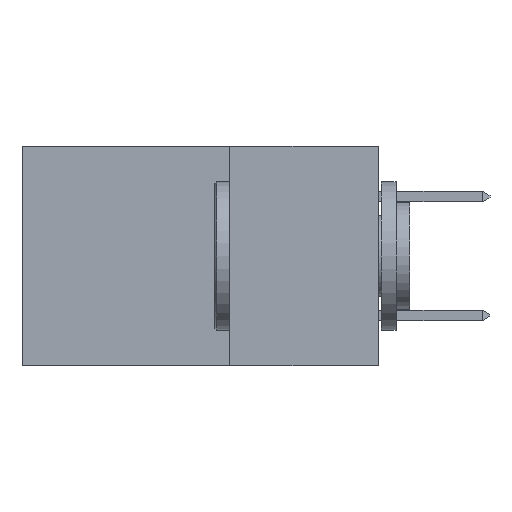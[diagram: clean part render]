
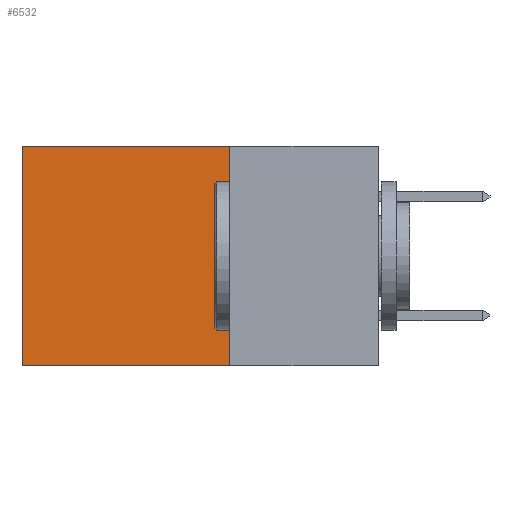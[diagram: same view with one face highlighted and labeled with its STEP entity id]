
A CAD part, left-side view. The second image highlights one B-rep face of the part: STEP entity #6532.
In plain terms, the highlighted planar face has unit normal (-1, 0, 0).
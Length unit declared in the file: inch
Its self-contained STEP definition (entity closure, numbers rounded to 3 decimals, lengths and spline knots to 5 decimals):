
#252 = LINE ( 'NONE', #10762, #7019 ) ;
#989 = EDGE_LOOP ( 'NONE', ( #15979, #15965, #16829, #6244 ) ) ;
#1613 = VERTEX_POINT ( 'NONE', #8101 ) ;
#2345 = LINE ( 'NONE', #16544, #5518 ) ;
#2947 = DIRECTION ( 'NONE',  ( 0., 0., -1. ) ) ;
#3176 = EDGE_CURVE ( 'NONE', #1613, #14830, #14307, .T. ) ;
#5518 = VECTOR ( 'NONE', #10008, 39.37008 ) ;
#5531 = VERTEX_POINT ( 'NONE', #16217 ) ;
#5588 = LINE ( 'NONE', #9181, #12341 ) ;
#5745 = CARTESIAN_POINT ( 'NONE',  ( 0.298, 0.25, -0.37 ) ) ;
#6244 = ORIENTED_EDGE ( 'NONE', *, *, #3176, .T. ) ;
#6532 = ADVANCED_FACE ( 'NONE', ( #12805 ), #8934, .F. ) ;
#7019 = VECTOR ( 'NONE', #14744, 39.37008 ) ;
#8101 = CARTESIAN_POINT ( 'NONE',  ( 0.298, 0.25, 0. ) ) ;
#8300 = AXIS2_PLACEMENT_3D ( 'NONE', #12078, #12023, #2947 ) ;
#8556 = EDGE_CURVE ( 'NONE', #15789, #5531, #252, .T. ) ;
#8934 = PLANE ( 'NONE',  #8300 ) ;
#9181 = CARTESIAN_POINT ( 'NONE',  ( 0.298, 0.6, 0. ) ) ;
#9912 = DIRECTION ( 'NONE',  ( 0., 1., 0. ) ) ;
#10008 = DIRECTION ( 'NONE',  ( 0., 0., -1. ) ) ;
#10762 = CARTESIAN_POINT ( 'NONE',  ( 0.298, 0.25, -0.37 ) ) ;
#10795 = VECTOR ( 'NONE', #9912, 39.37008 ) ;
#11926 = DIRECTION ( 'NONE',  ( 0., 0., -1. ) ) ;
#12023 = DIRECTION ( 'NONE',  ( 1., 0., 0. ) ) ;
#12078 = CARTESIAN_POINT ( 'NONE',  ( 0.298, 0.25, 0. ) ) ;
#12341 = VECTOR ( 'NONE', #11926, 39.37008 ) ;
#12805 = FACE_OUTER_BOUND ( 'NONE', #989, .T. ) ;
#12824 = EDGE_CURVE ( 'NONE', #14830, #5531, #5588, .T. ) ;
#14302 = CARTESIAN_POINT ( 'NONE',  ( 0.298, 0.25, 0. ) ) ;
#14307 = LINE ( 'NONE', #14302, #10795 ) ;
#14744 = DIRECTION ( 'NONE',  ( 0., 1., 0. ) ) ;
#14830 = VERTEX_POINT ( 'NONE', #15880 ) ;
#15182 = EDGE_CURVE ( 'NONE', #1613, #15789, #2345, .T. ) ;
#15789 = VERTEX_POINT ( 'NONE', #5745 ) ;
#15880 = CARTESIAN_POINT ( 'NONE',  ( 0.298, 0.6, 0. ) ) ;
#15965 = ORIENTED_EDGE ( 'NONE', *, *, #8556, .F. ) ;
#15979 = ORIENTED_EDGE ( 'NONE', *, *, #12824, .T. ) ;
#16217 = CARTESIAN_POINT ( 'NONE',  ( 0.298, 0.6, -0.37 ) ) ;
#16544 = CARTESIAN_POINT ( 'NONE',  ( 0.298, 0.25, 0. ) ) ;
#16829 = ORIENTED_EDGE ( 'NONE', *, *, #15182, .F. ) ;
